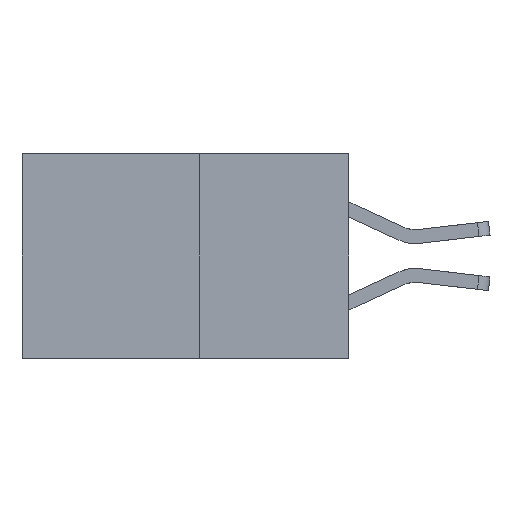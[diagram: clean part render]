
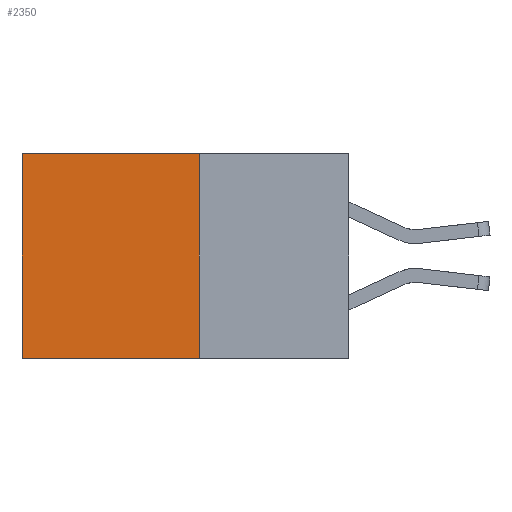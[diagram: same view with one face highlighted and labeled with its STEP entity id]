
A CAD part, left-side view. The second image highlights one B-rep face of the part: STEP entity #2350.
In plain terms, the highlighted planar face has unit normal (-1, 0, 0).
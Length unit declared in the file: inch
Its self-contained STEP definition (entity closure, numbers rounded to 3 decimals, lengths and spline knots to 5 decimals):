
#226 = DIRECTION ( 'NONE',  ( 0., 0., -1. ) ) ;
#788 = LINE ( 'NONE', #5890, #8709 ) ;
#1084 = DIRECTION ( 'NONE',  ( 0., 1., 0. ) ) ;
#1331 = CARTESIAN_POINT ( 'NONE',  ( 0.277, 0.27, -0.37 ) ) ;
#1414 = CARTESIAN_POINT ( 'NONE',  ( 0.277, 0.59, -0.37 ) ) ;
#1754 = EDGE_CURVE ( 'NONE', #6997, #8790, #3134, .T. ) ;
#2113 = FACE_OUTER_BOUND ( 'NONE', #10217, .T. ) ;
#2350 = ADVANCED_FACE ( 'NONE', ( #2113 ), #5533, .F. ) ;
#2354 = AXIS2_PLACEMENT_3D ( 'NONE', #5603, #5502, #7551 ) ;
#2798 = CARTESIAN_POINT ( 'NONE',  ( 0.277, 0.27, -0.37 ) ) ;
#2886 = VECTOR ( 'NONE', #8055, 39.37008 ) ;
#2923 = ORIENTED_EDGE ( 'NONE', *, *, #9932, .T. ) ;
#3134 = LINE ( 'NONE', #8076, #2886 ) ;
#3173 = ORIENTED_EDGE ( 'NONE', *, *, #8010, .F. ) ;
#3416 = ORIENTED_EDGE ( 'NONE', *, *, #1754, .T. ) ;
#3471 = EDGE_CURVE ( 'NONE', #6500, #6739, #8689, .T. ) ;
#4062 = DIRECTION ( 'NONE',  ( 0., 0., -1. ) ) ;
#4460 = VECTOR ( 'NONE', #4062, 39.37008 ) ;
#4894 = CARTESIAN_POINT ( 'NONE',  ( 0.277, 0.27, 0. ) ) ;
#4999 = ORIENTED_EDGE ( 'NONE', *, *, #3471, .F. ) ;
#5502 = DIRECTION ( 'NONE',  ( 1., 0., 0. ) ) ;
#5533 = PLANE ( 'NONE',  #2354 ) ;
#5603 = CARTESIAN_POINT ( 'NONE',  ( 0.277, 0.27, -0.37 ) ) ;
#5875 = CARTESIAN_POINT ( 'NONE',  ( 0.277, 0.59, 0. ) ) ;
#5890 = CARTESIAN_POINT ( 'NONE',  ( 0.277, 0.59, -0.37 ) ) ;
#6064 = LINE ( 'NONE', #8701, #4460 ) ;
#6186 = VECTOR ( 'NONE', #1084, 39.37008 ) ;
#6500 = VERTEX_POINT ( 'NONE', #2798 ) ;
#6739 = VERTEX_POINT ( 'NONE', #1414 ) ;
#6997 = VERTEX_POINT ( 'NONE', #4894 ) ;
#7551 = DIRECTION ( 'NONE',  ( 0., 0., -1. ) ) ;
#8010 = EDGE_CURVE ( 'NONE', #6997, #6500, #6064, .T. ) ;
#8055 = DIRECTION ( 'NONE',  ( 0., 1., 0. ) ) ;
#8076 = CARTESIAN_POINT ( 'NONE',  ( 0.277, 0.27, 0. ) ) ;
#8689 = LINE ( 'NONE', #1331, #6186 ) ;
#8701 = CARTESIAN_POINT ( 'NONE',  ( 0.277, 0.27, -0.37 ) ) ;
#8709 = VECTOR ( 'NONE', #226, 39.37008 ) ;
#8790 = VERTEX_POINT ( 'NONE', #5875 ) ;
#9932 = EDGE_CURVE ( 'NONE', #8790, #6739, #788, .T. ) ;
#10217 = EDGE_LOOP ( 'NONE', ( #2923, #4999, #3173, #3416 ) ) ;
